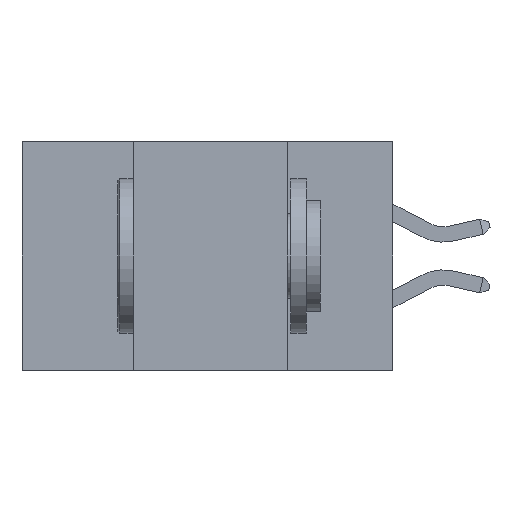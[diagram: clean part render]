
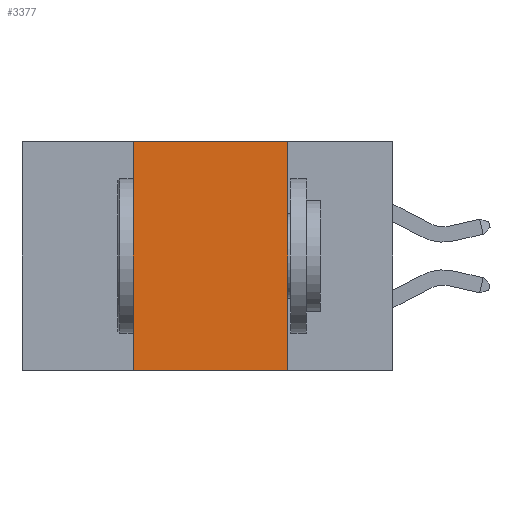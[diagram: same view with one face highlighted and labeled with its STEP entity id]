
A CAD part, left-side view. The second image highlights one B-rep face of the part: STEP entity #3377.
In plain terms, the highlighted planar face has unit normal (-1, 0, 0).
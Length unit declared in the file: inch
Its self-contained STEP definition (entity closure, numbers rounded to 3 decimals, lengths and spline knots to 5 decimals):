
#57 = CARTESIAN_POINT ( 'NONE',  ( 0., 0.42, 0. ) ) ;
#566 = LINE ( 'NONE', #4099, #2429 ) ;
#640 = EDGE_CURVE ( 'NONE', #1569, #7113, #566, .T. ) ;
#1004 = VERTEX_POINT ( 'NONE', #6879 ) ;
#1377 = LINE ( 'NONE', #6872, #3205 ) ;
#1569 = VERTEX_POINT ( 'NONE', #57 ) ;
#1820 = ORIENTED_EDGE ( 'NONE', *, *, #2971, .F. ) ;
#1831 = ORIENTED_EDGE ( 'NONE', *, *, #640, .F. ) ;
#2296 = ORIENTED_EDGE ( 'NONE', *, *, #3092, .F. ) ;
#2313 = ORIENTED_EDGE ( 'NONE', *, *, #2822, .T. ) ;
#2429 = VECTOR ( 'NONE', #9652, 39.37008 ) ;
#2822 = EDGE_CURVE ( 'NONE', #1004, #8135, #3574, .T. ) ;
#2971 = EDGE_CURVE ( 'NONE', #7113, #8135, #6523, .T. ) ;
#3092 = EDGE_CURVE ( 'NONE', #1004, #1569, #1377, .T. ) ;
#3205 = VECTOR ( 'NONE', #6885, 39.37008 ) ;
#3377 = ADVANCED_FACE ( 'NONE', ( #5057 ), #5196, .F. ) ;
#3574 = LINE ( 'NONE', #8809, #9442 ) ;
#4099 = CARTESIAN_POINT ( 'NONE',  ( 0., 0.6, 0. ) ) ;
#4175 = VECTOR ( 'NONE', #7653, 39.37008 ) ;
#5057 = FACE_OUTER_BOUND ( 'NONE', #6441, .T. ) ;
#5110 = DIRECTION ( 'NONE',  ( 0., 0., -1. ) ) ;
#5111 = DIRECTION ( 'NONE',  ( 1., 0., 0. ) ) ;
#5131 = CARTESIAN_POINT ( 'NONE',  ( 0., 0.6, 0. ) ) ;
#5196 = PLANE ( 'NONE',  #5417 ) ;
#5417 = AXIS2_PLACEMENT_3D ( 'NONE', #5131, #5111, #5110 ) ;
#5944 = CARTESIAN_POINT ( 'NONE',  ( 0., 0.17, -0.37 ) ) ;
#6441 = EDGE_LOOP ( 'NONE', ( #1820, #1831, #2296, #2313 ) ) ;
#6523 = LINE ( 'NONE', #7663, #4175 ) ;
#6872 = CARTESIAN_POINT ( 'NONE',  ( 0., 0.42, 0. ) ) ;
#6879 = CARTESIAN_POINT ( 'NONE',  ( 0., 0.42, -0.37 ) ) ;
#6885 = DIRECTION ( 'NONE',  ( 0., 0., 1. ) ) ;
#6935 = CARTESIAN_POINT ( 'NONE',  ( 0., 0.17, 0. ) ) ;
#7113 = VERTEX_POINT ( 'NONE', #6935 ) ;
#7653 = DIRECTION ( 'NONE',  ( 0., 0., -1. ) ) ;
#7663 = CARTESIAN_POINT ( 'NONE',  ( 0., 0.17, 0. ) ) ;
#8135 = VERTEX_POINT ( 'NONE', #5944 ) ;
#8653 = DIRECTION ( 'NONE',  ( 0., -1., 0. ) ) ;
#8809 = CARTESIAN_POINT ( 'NONE',  ( 0., 0.6, -0.37 ) ) ;
#9442 = VECTOR ( 'NONE', #8653, 39.37008 ) ;
#9652 = DIRECTION ( 'NONE',  ( 0., -1., 0. ) ) ;
